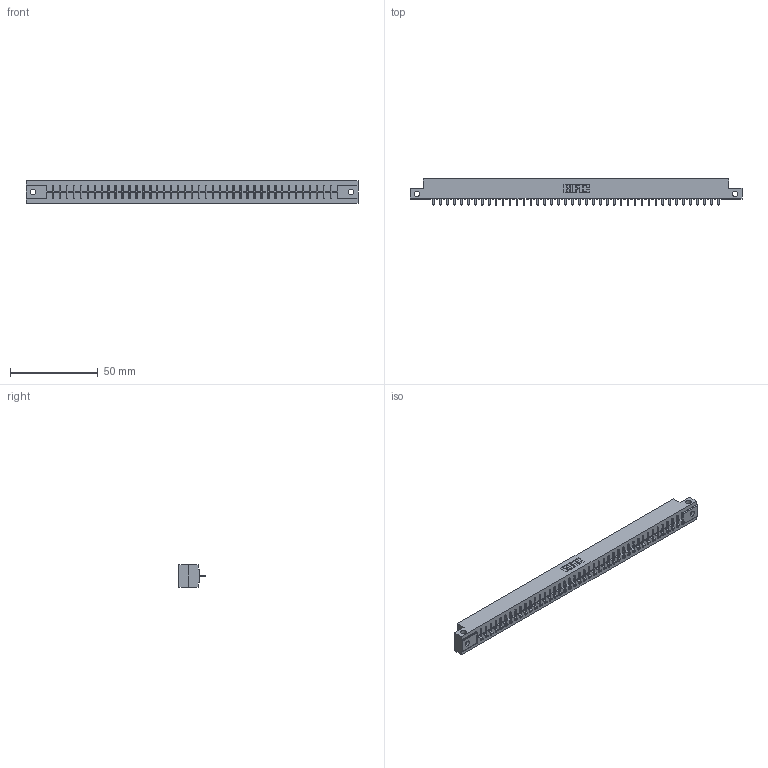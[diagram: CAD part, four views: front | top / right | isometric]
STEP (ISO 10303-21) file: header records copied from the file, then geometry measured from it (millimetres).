
FILE_DESCRIPTION (( 'STEP AP203' ), '1' );
FILE_NAME ('316-042-421-112.STEP', '2020-09-23T07:44:16', ( '' ), ( '' ), 'SwSTEP 2.0', 'SolidWorks 2020', '' );
FILE_SCHEMA (( 'CONFIG_CONTROL_DESIGN' ));
Length unit declared in the file: inch
Products named in the file (3): 316-042-421-112; 306-290-001_121; 306 Part_.128 Dia
Assembly tree (43 placements, depth 2):
  316-042-421-112
    306 Part_.128 Dia
    306-290-001_121  x42
Bounding box: 189.43 x 14.88 x 12.7 mm (x, y, z)
Volume: 20701.7 mm3; surface area: 20964.3 mm2
Topology: 43 solids, 43 shells, 3068 faces, 8626 edges, 5520 vertices
Faces by surface type: plane 2042, cylinder 858, sphere 168
Entity records: 39529 total; most frequent: CARTESIAN_POINT 6685, ORIENTED_EDGE 6584, DIRECTION 6530, EDGE_CURVE 3292, VECTOR 2560, LINE 2560, VERTEX_POINT 2076, AXIS2_PLACEMENT_3D 1985
